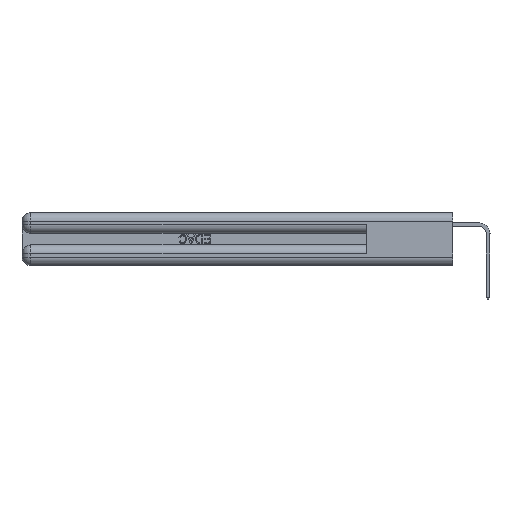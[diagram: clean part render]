
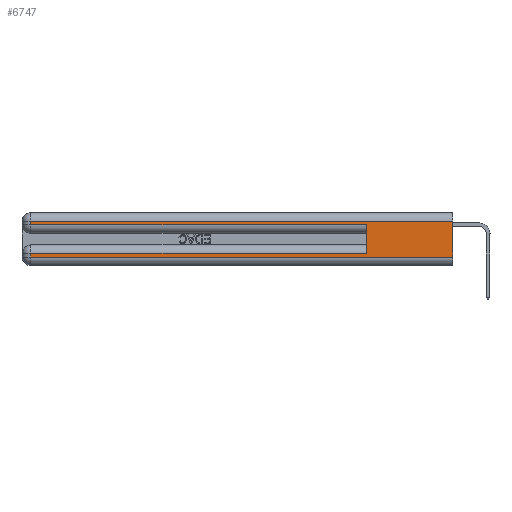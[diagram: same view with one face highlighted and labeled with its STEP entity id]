
A CAD part, left-side view. The second image highlights one B-rep face of the part: STEP entity #6747.
In plain terms, the highlighted planar face has unit normal (-1, 0, 0).
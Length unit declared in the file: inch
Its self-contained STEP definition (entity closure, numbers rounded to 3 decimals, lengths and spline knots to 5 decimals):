
#91 = DIRECTION ( 'NONE',  ( 0., 0., -1. ) ) ;
#1505 = VERTEX_POINT ( 'NONE', #21775 ) ;
#2561 = VERTEX_POINT ( 'NONE', #36506 ) ;
#2641 = CARTESIAN_POINT ( 'NONE',  ( 0., 0., 0.06 ) ) ;
#3044 = LINE ( 'NONE', #26250, #35985 ) ;
#3674 = LINE ( 'NONE', #9254, #15856 ) ;
#5462 = EDGE_CURVE ( 'NONE', #39521, #28839, #30229, .T. ) ;
#5982 = CARTESIAN_POINT ( 'NONE',  ( 0., 2.94, 0.31 ) ) ;
#6018 = CARTESIAN_POINT ( 'NONE',  ( 0., 2.94, 0.285 ) ) ;
#6146 = VECTOR ( 'NONE', #32436, 39.37008 ) ;
#6456 = CARTESIAN_POINT ( 'NONE',  ( 0., 0., 0.06 ) ) ;
#6520 = LINE ( 'NONE', #38397, #22630 ) ;
#6714 = VERTEX_POINT ( 'NONE', #11909 ) ;
#6747 = ADVANCED_FACE ( 'NONE', ( #8765 ), #24844, .F. ) ;
#8765 = FACE_OUTER_BOUND ( 'NONE', #17754, .T. ) ;
#8898 = CARTESIAN_POINT ( 'NONE',  ( 0., 2.94, 0.085 ) ) ;
#9254 = CARTESIAN_POINT ( 'NONE',  ( 0., 0.6, 0.145 ) ) ;
#10959 = EDGE_CURVE ( 'NONE', #39521, #17881, #25684, .T. ) ;
#11909 = CARTESIAN_POINT ( 'NONE',  ( 0., 0.6, 0.285 ) ) ;
#12291 = EDGE_CURVE ( 'NONE', #17881, #20387, #6520, .T. ) ;
#13448 = ORIENTED_EDGE ( 'NONE', *, *, #5462, .F. ) ;
#14366 = ORIENTED_EDGE ( 'NONE', *, *, #10959, .T. ) ;
#14409 = ORIENTED_EDGE ( 'NONE', *, *, #12291, .T. ) ;
#14446 = EDGE_CURVE ( 'NONE', #20387, #6714, #38086, .T. ) ;
#14806 = ORIENTED_EDGE ( 'NONE', *, *, #14446, .T. ) ;
#14923 = ORIENTED_EDGE ( 'NONE', *, *, #15233, .F. ) ;
#15233 = EDGE_CURVE ( 'NONE', #2561, #6714, #3674, .T. ) ;
#15283 = ORIENTED_EDGE ( 'NONE', *, *, #16843, .T. ) ;
#15856 = VECTOR ( 'NONE', #28285, 39.37008 ) ;
#16080 = CARTESIAN_POINT ( 'NONE',  ( 0., 0., 0.31 ) ) ;
#16222 = ORIENTED_EDGE ( 'NONE', *, *, #19332, .T. ) ;
#16253 = VECTOR ( 'NONE', #25644, 39.37008 ) ;
#16298 = ORIENTED_EDGE ( 'NONE', *, *, #23784, .T. ) ;
#16588 = CARTESIAN_POINT ( 'NONE',  ( 0., 2.94, 0.37 ) ) ;
#16832 = DIRECTION ( 'NONE',  ( 0., 1., 0. ) ) ;
#16843 = EDGE_CURVE ( 'NONE', #2561, #20940, #3044, .T. ) ;
#17754 = EDGE_LOOP ( 'NONE', ( #13448, #14366, #14409, #14806, #14923, #15283, #16222, #16298 ) ) ;
#17881 = VERTEX_POINT ( 'NONE', #5982 ) ;
#18484 = DIRECTION ( 'NONE',  ( 0., 0., -1. ) ) ;
#19332 = EDGE_CURVE ( 'NONE', #20940, #1505, #23268, .T. ) ;
#20017 = LINE ( 'NONE', #6456, #35687 ) ;
#20387 = VERTEX_POINT ( 'NONE', #6018 ) ;
#20940 = VERTEX_POINT ( 'NONE', #8898 ) ;
#21713 = CARTESIAN_POINT ( 'NONE',  ( 0., 0., 0.37 ) ) ;
#21775 = CARTESIAN_POINT ( 'NONE',  ( 0., 2.94, 0.06 ) ) ;
#22443 = VECTOR ( 'NONE', #33539, 39.37008 ) ;
#22630 = VECTOR ( 'NONE', #91, 39.37008 ) ;
#23268 = LINE ( 'NONE', #16588, #6146 ) ;
#23784 = EDGE_CURVE ( 'NONE', #1505, #28839, #20017, .T. ) ;
#23833 = CARTESIAN_POINT ( 'NONE',  ( 0., 0., 0.31 ) ) ;
#24225 = CARTESIAN_POINT ( 'NONE',  ( 0., 0., 0.285 ) ) ;
#24844 = PLANE ( 'NONE',  #36812 ) ;
#25505 = DIRECTION ( 'NONE',  ( 0., -1., 0. ) ) ;
#25644 = DIRECTION ( 'NONE',  ( 0., 1., 0. ) ) ;
#25684 = LINE ( 'NONE', #16080, #16253 ) ;
#26250 = CARTESIAN_POINT ( 'NONE',  ( 0., 0., 0.085 ) ) ;
#27850 = CARTESIAN_POINT ( 'NONE',  ( 0., 0., 0.37 ) ) ;
#28023 = DIRECTION ( 'NONE',  ( 0., 0., -1. ) ) ;
#28285 = DIRECTION ( 'NONE',  ( 0., 0., 1. ) ) ;
#28839 = VERTEX_POINT ( 'NONE', #2641 ) ;
#30229 = LINE ( 'NONE', #27850, #37561 ) ;
#31019 = DIRECTION ( 'NONE',  ( 1., 0., 0. ) ) ;
#32436 = DIRECTION ( 'NONE',  ( 0., 0., -1. ) ) ;
#33539 = DIRECTION ( 'NONE',  ( 0., -1., 0. ) ) ;
#35687 = VECTOR ( 'NONE', #25505, 39.37008 ) ;
#35985 = VECTOR ( 'NONE', #16832, 39.37008 ) ;
#36506 = CARTESIAN_POINT ( 'NONE',  ( 0., 0.6, 0.085 ) ) ;
#36812 = AXIS2_PLACEMENT_3D ( 'NONE', #21713, #31019, #28023 ) ;
#37561 = VECTOR ( 'NONE', #18484, 39.37008 ) ;
#38086 = LINE ( 'NONE', #24225, #22443 ) ;
#38397 = CARTESIAN_POINT ( 'NONE',  ( 0., 2.94, 0.37 ) ) ;
#39521 = VERTEX_POINT ( 'NONE', #23833 ) ;
